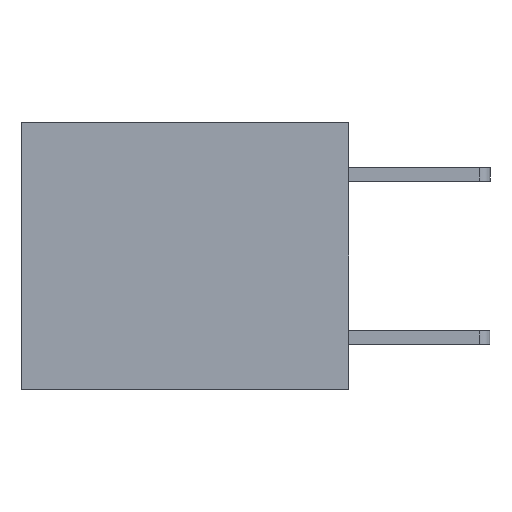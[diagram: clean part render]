
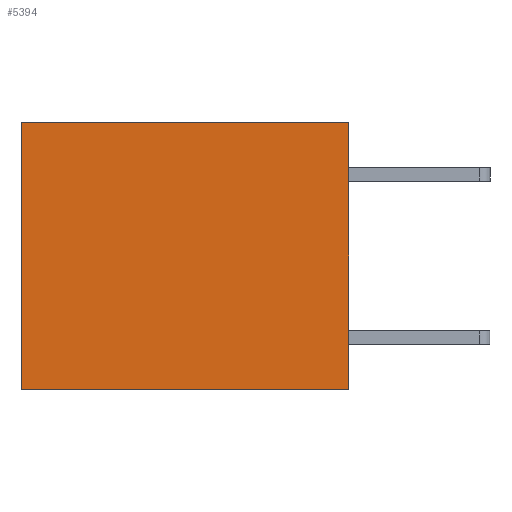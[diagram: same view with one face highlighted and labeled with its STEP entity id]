
A CAD part, left-side view. The second image highlights one B-rep face of the part: STEP entity #5394.
In plain terms, the highlighted planar face has unit normal (-1, 0, 0).
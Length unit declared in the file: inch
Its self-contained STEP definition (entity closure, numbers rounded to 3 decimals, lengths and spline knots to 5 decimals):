
#159 = CARTESIAN_POINT ( 'NONE',  ( 0.3165, 0., -0.49 ) ) ;
#370 = LINE ( 'NONE', #6910, #5398 ) ;
#528 = DIRECTION ( 'NONE',  ( 1., 0., 0. ) ) ;
#598 = ORIENTED_EDGE ( 'NONE', *, *, #6979, .T. ) ;
#1514 = CARTESIAN_POINT ( 'NONE',  ( 0.3165, 0., 0. ) ) ;
#1679 = VECTOR ( 'NONE', #2506, 39.37008 ) ;
#1997 = DIRECTION ( 'NONE',  ( 0., 0., -1. ) ) ;
#2050 = CARTESIAN_POINT ( 'NONE',  ( 0.3165, 0.6, 0. ) ) ;
#2210 = VECTOR ( 'NONE', #1997, 39.37008 ) ;
#2506 = DIRECTION ( 'NONE',  ( 0., 0., -1. ) ) ;
#2636 = DIRECTION ( 'NONE',  ( 0., 0., -1. ) ) ;
#2665 = CARTESIAN_POINT ( 'NONE',  ( 0.3165, 0., -0.49 ) ) ;
#3541 = VERTEX_POINT ( 'NONE', #6533 ) ;
#3731 = VECTOR ( 'NONE', #6717, 39.37008 ) ;
#3852 = DIRECTION ( 'NONE',  ( 0., 1., 0. ) ) ;
#4017 = EDGE_CURVE ( 'NONE', #3541, #8225, #6652, .T. ) ;
#4117 = EDGE_LOOP ( 'NONE', ( #598, #7035, #4585, #8781 ) ) ;
#4315 = CARTESIAN_POINT ( 'NONE',  ( 0.3165, 0., -0.49 ) ) ;
#4585 = ORIENTED_EDGE ( 'NONE', *, *, #4017, .F. ) ;
#4896 = LINE ( 'NONE', #1514, #3731 ) ;
#4969 = LINE ( 'NONE', #9232, #1679 ) ;
#5087 = EDGE_CURVE ( 'NONE', #3541, #7112, #4896, .T. ) ;
#5394 = ADVANCED_FACE ( 'NONE', ( #7322 ), #8732, .F. ) ;
#5398 = VECTOR ( 'NONE', #3852, 39.37008 ) ;
#6351 = VERTEX_POINT ( 'NONE', #8621 ) ;
#6533 = CARTESIAN_POINT ( 'NONE',  ( 0.3165, 0., 0. ) ) ;
#6652 = LINE ( 'NONE', #4315, #2210 ) ;
#6717 = DIRECTION ( 'NONE',  ( 0., 1., 0. ) ) ;
#6910 = CARTESIAN_POINT ( 'NONE',  ( 0.3165, 0., -0.49 ) ) ;
#6979 = EDGE_CURVE ( 'NONE', #7112, #6351, #4969, .T. ) ;
#7035 = ORIENTED_EDGE ( 'NONE', *, *, #9663, .F. ) ;
#7112 = VERTEX_POINT ( 'NONE', #2050 ) ;
#7322 = FACE_OUTER_BOUND ( 'NONE', #4117, .T. ) ;
#7801 = AXIS2_PLACEMENT_3D ( 'NONE', #2665, #528, #2636 ) ;
#8225 = VERTEX_POINT ( 'NONE', #159 ) ;
#8621 = CARTESIAN_POINT ( 'NONE',  ( 0.3165, 0.6, -0.49 ) ) ;
#8732 = PLANE ( 'NONE',  #7801 ) ;
#8781 = ORIENTED_EDGE ( 'NONE', *, *, #5087, .T. ) ;
#9232 = CARTESIAN_POINT ( 'NONE',  ( 0.3165, 0.6, -0.49 ) ) ;
#9663 = EDGE_CURVE ( 'NONE', #8225, #6351, #370, .T. ) ;
